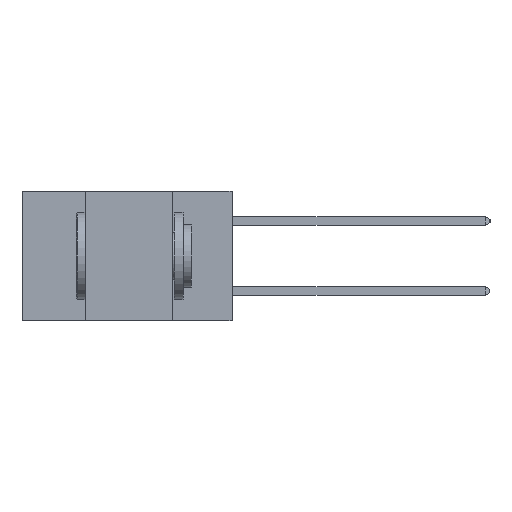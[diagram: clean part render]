
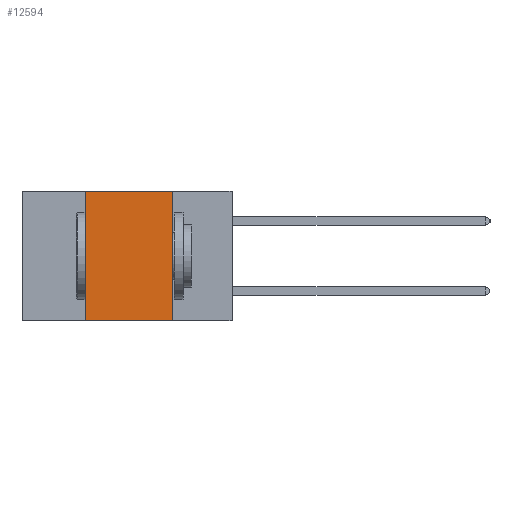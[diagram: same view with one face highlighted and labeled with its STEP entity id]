
A CAD part, left-side view. The second image highlights one B-rep face of the part: STEP entity #12594.
In plain terms, the highlighted planar face has unit normal (-1, 0, 0).
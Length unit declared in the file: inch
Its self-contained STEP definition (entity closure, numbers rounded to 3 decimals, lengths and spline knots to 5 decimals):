
#509 = CARTESIAN_POINT ( 'NONE',  ( 0., 0.17, 0. ) ) ;
#987 = ORIENTED_EDGE ( 'NONE', *, *, #21956, .F. ) ;
#1129 = LINE ( 'NONE', #17721, #15106 ) ;
#1851 = ORIENTED_EDGE ( 'NONE', *, *, #9404, .T. ) ;
#2241 = PLANE ( 'NONE',  #20728 ) ;
#2367 = DIRECTION ( 'NONE',  ( 0., 0., -1. ) ) ;
#3964 = VECTOR ( 'NONE', #2367, 39.37008 ) ;
#4032 = FACE_OUTER_BOUND ( 'NONE', #5603, .T. ) ;
#4153 = DIRECTION ( 'NONE',  ( 0., 0., -1. ) ) ;
#5328 = CARTESIAN_POINT ( 'NONE',  ( 0., 0.42, 0. ) ) ;
#5603 = EDGE_LOOP ( 'NONE', ( #20070, #12110, #987, #1851 ) ) ;
#6289 = VERTEX_POINT ( 'NONE', #5328 ) ;
#7035 = VECTOR ( 'NONE', #19900, 39.37008 ) ;
#7637 = VERTEX_POINT ( 'NONE', #21674 ) ;
#8813 = EDGE_CURVE ( 'NONE', #6289, #19744, #1129, .T. ) ;
#8817 = CARTESIAN_POINT ( 'NONE',  ( 0., 0.42, 0. ) ) ;
#9404 = EDGE_CURVE ( 'NONE', #7637, #20662, #11295, .T. ) ;
#9449 = CARTESIAN_POINT ( 'NONE',  ( 0., 0.6, -0.37 ) ) ;
#9560 = LINE ( 'NONE', #509, #3964 ) ;
#10728 = EDGE_CURVE ( 'NONE', #19744, #20662, #9560, .T. ) ;
#10951 = VECTOR ( 'NONE', #21026, 39.37008 ) ;
#11295 = LINE ( 'NONE', #9449, #7035 ) ;
#12110 = ORIENTED_EDGE ( 'NONE', *, *, #8813, .F. ) ;
#12594 = ADVANCED_FACE ( 'NONE', ( #4032 ), #2241, .F. ) ;
#14114 = CARTESIAN_POINT ( 'NONE',  ( 0., 0.17, -0.37 ) ) ;
#14977 = DIRECTION ( 'NONE',  ( 1., 0., 0. ) ) ;
#15106 = VECTOR ( 'NONE', #15966, 39.37008 ) ;
#15395 = CARTESIAN_POINT ( 'NONE',  ( 0., 0.17, 0. ) ) ;
#15966 = DIRECTION ( 'NONE',  ( 0., -1., 0. ) ) ;
#16655 = CARTESIAN_POINT ( 'NONE',  ( 0., 0.6, 0. ) ) ;
#17721 = CARTESIAN_POINT ( 'NONE',  ( 0., 0.6, 0. ) ) ;
#19744 = VERTEX_POINT ( 'NONE', #15395 ) ;
#19900 = DIRECTION ( 'NONE',  ( 0., -1., 0. ) ) ;
#20070 = ORIENTED_EDGE ( 'NONE', *, *, #10728, .F. ) ;
#20209 = LINE ( 'NONE', #8817, #10951 ) ;
#20662 = VERTEX_POINT ( 'NONE', #14114 ) ;
#20728 = AXIS2_PLACEMENT_3D ( 'NONE', #16655, #14977, #4153 ) ;
#21026 = DIRECTION ( 'NONE',  ( 0., 0., 1. ) ) ;
#21674 = CARTESIAN_POINT ( 'NONE',  ( 0., 0.42, -0.37 ) ) ;
#21956 = EDGE_CURVE ( 'NONE', #7637, #6289, #20209, .T. ) ;
